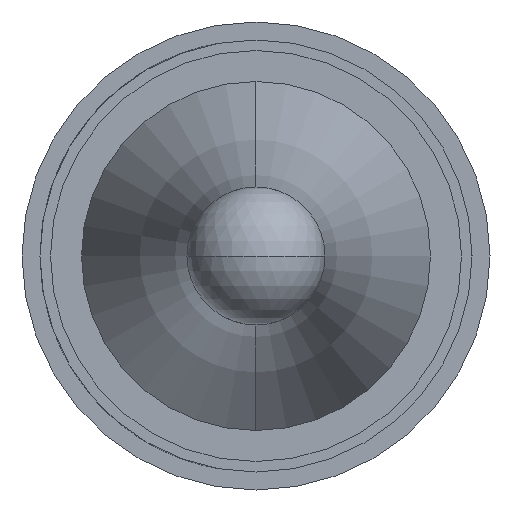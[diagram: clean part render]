
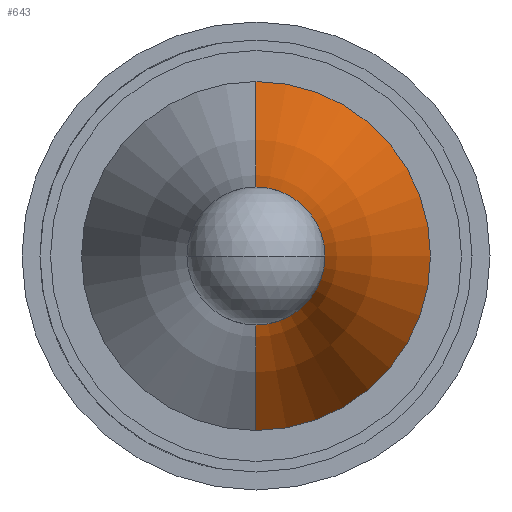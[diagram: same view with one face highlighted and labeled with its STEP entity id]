
A CAD part, left-side view. The second image highlights one B-rep face of the part: STEP entity #643.
In plain terms, the highlighted toroidal (fillet/blend) face has major radius 15.646 mm and minor radius 14.77 mm.
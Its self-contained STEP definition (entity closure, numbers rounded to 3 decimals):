
#38 = DIRECTION ( 'NONE',  ( 0., 0., -1. ) ) ;
#43 = DIRECTION ( 'NONE',  ( 1., 0., 0. ) ) ;
#46 = CARTESIAN_POINT ( 'NONE',  ( -41.846, 0., 0. ) ) ;
#113 = ORIENTED_EDGE ( 'NONE', *, *, #702, .T. ) ;
#140 = AXIS2_PLACEMENT_3D ( 'NONE', #428, #365, #359 ) ;
#141 = AXIS2_PLACEMENT_3D ( 'NONE', #504, #498, #452 ) ;
#144 = VERTEX_POINT ( 'NONE', #943 ) ;
#145 = AXIS2_PLACEMENT_3D ( 'NONE', #614, #589, #583 ) ;
#149 = AXIS2_PLACEMENT_3D ( 'NONE', #689, #666, #664 ) ;
#161 = AXIS2_PLACEMENT_3D ( 'NONE', #772, #766, #749 ) ;
#169 = AXIS2_PLACEMENT_3D ( 'NONE', #46, #43, #38 ) ;
#187 = AXIS2_PLACEMENT_3D ( 'NONE', #375, #370, #353 ) ;
#209 = EDGE_LOOP ( 'NONE', ( #267, #113, #245, #480, #710, #910 ) ) ;
#222 = VERTEX_POINT ( 'NONE', #281 ) ;
#245 = ORIENTED_EDGE ( 'NONE', *, *, #707, .T. ) ;
#267 = ORIENTED_EDGE ( 'NONE', *, *, #675, .F. ) ;
#281 = CARTESIAN_POINT ( 'NONE',  ( -41.846, 0., 2.216 ) ) ;
#353 = DIRECTION ( 'NONE',  ( 0., 0., -1. ) ) ;
#359 = DIRECTION ( 'NONE',  ( 0., 0., -1. ) ) ;
#365 = DIRECTION ( 'NONE',  ( 1., 0., 0. ) ) ;
#370 = DIRECTION ( 'NONE',  ( 1., 0., 0. ) ) ;
#375 = CARTESIAN_POINT ( 'NONE',  ( -47.993, 0., 0. ) ) ;
#396 = CIRCLE ( 'NONE', #141, 14.77 ) ;
#397 = CARTESIAN_POINT ( 'NONE',  ( -47.993, 0., -0.876 ) ) ;
#406 = CARTESIAN_POINT ( 'NONE',  ( -41.846, -2.216, 0. ) ) ;
#428 = CARTESIAN_POINT ( 'NONE',  ( -41.846, 0., 0. ) ) ;
#452 = DIRECTION ( 'NONE',  ( 0., 0., -1. ) ) ;
#480 = ORIENTED_EDGE ( 'NONE', *, *, #714, .T. ) ;
#491 = FACE_OUTER_BOUND ( 'NONE', #209, .T. ) ;
#498 = DIRECTION ( 'NONE',  ( 0., -1., 0. ) ) ;
#504 = CARTESIAN_POINT ( 'NONE',  ( -47.993, 0., -15.646 ) ) ;
#530 = VERTEX_POINT ( 'NONE', #397 ) ;
#540 = VERTEX_POINT ( 'NONE', #406 ) ;
#583 = DIRECTION ( 'NONE',  ( 0., 0., -1. ) ) ;
#589 = DIRECTION ( 'NONE',  ( 1., 0., 0. ) ) ;
#602 = CARTESIAN_POINT ( 'NONE',  ( -47.993, -0.876, 0. ) ) ;
#614 = CARTESIAN_POINT ( 'NONE',  ( -47.993, 0., 0. ) ) ;
#618 = CIRCLE ( 'NONE', #145, 0.876 ) ;
#643 = ADVANCED_FACE ( 'NONE', ( #491 ), #711, .F. ) ;
#664 = DIRECTION ( 'NONE',  ( 0., 0., -1. ) ) ;
#666 = DIRECTION ( 'NONE',  ( 1., 0., 0. ) ) ;
#675 = EDGE_CURVE ( 'NONE', #222, #540, #871, .T. ) ;
#689 = CARTESIAN_POINT ( 'NONE',  ( -47.993, 0., 0. ) ) ;
#702 = EDGE_CURVE ( 'NONE', #222, #144, #850, .T. ) ;
#707 = EDGE_CURVE ( 'NONE', #144, #862, #1016, .T. ) ;
#710 = ORIENTED_EDGE ( 'NONE', *, *, #716, .F. ) ;
#711 = TOROIDAL_SURFACE ( 'NONE', #187, 15.646, 14.77 ) ;
#714 = EDGE_CURVE ( 'NONE', #862, #530, #618, .T. ) ;
#716 = EDGE_CURVE ( 'NONE', #1023, #530, #396, .T. ) ;
#723 = EDGE_CURVE ( 'NONE', #540, #1023, #825, .T. ) ;
#749 = DIRECTION ( 'NONE',  ( 0., 0., 1. ) ) ;
#766 = DIRECTION ( 'NONE',  ( 0., 1., 0. ) ) ;
#772 = CARTESIAN_POINT ( 'NONE',  ( -47.993, 0., 15.646 ) ) ;
#825 = CIRCLE ( 'NONE', #140, 2.216 ) ;
#850 = CIRCLE ( 'NONE', #161, 14.77 ) ;
#862 = VERTEX_POINT ( 'NONE', #602 ) ;
#871 = CIRCLE ( 'NONE', #169, 2.216 ) ;
#910 = ORIENTED_EDGE ( 'NONE', *, *, #723, .F. ) ;
#943 = CARTESIAN_POINT ( 'NONE',  ( -47.993, 0., 0.876 ) ) ;
#1016 = CIRCLE ( 'NONE', #149, 0.876 ) ;
#1023 = VERTEX_POINT ( 'NONE', #1083 ) ;
#1083 = CARTESIAN_POINT ( 'NONE',  ( -41.846, 0., -2.216 ) ) ;
